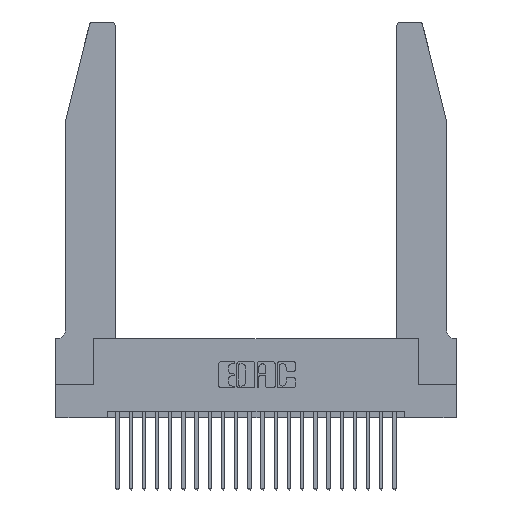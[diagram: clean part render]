
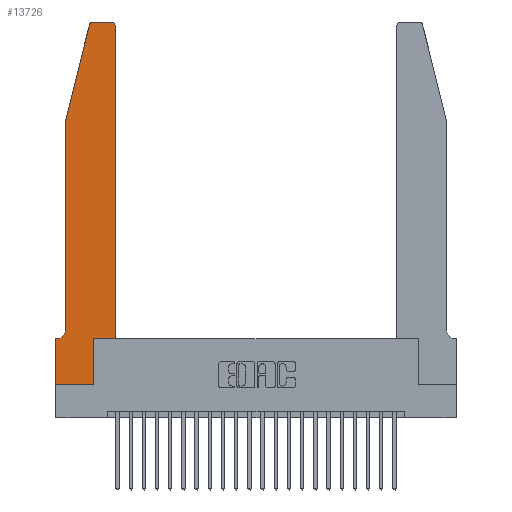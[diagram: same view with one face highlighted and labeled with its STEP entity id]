
A CAD part, top view. The second image highlights one B-rep face of the part: STEP entity #13726.
In plain terms, the highlighted planar face has unit normal (0, 0, 1).
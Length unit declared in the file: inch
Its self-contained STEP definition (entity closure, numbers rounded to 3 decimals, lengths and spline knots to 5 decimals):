
#131 = CARTESIAN_POINT ( 'NONE',  ( 0.0755, 2., 0.37 ) ) ;
#181 = CARTESIAN_POINT ( 'NONE',  ( 0., 0.35, 0.37 ) ) ;
#459 = DIRECTION ( 'NONE',  ( -1., 0., 0. ) ) ;
#518 = CARTESIAN_POINT ( 'NONE',  ( 0.0755, 2., 0.37 ) ) ;
#807 = VERTEX_POINT ( 'NONE', #22162 ) ;
#1023 = LINE ( 'NONE', #17720, #10701 ) ;
#1210 = VERTEX_POINT ( 'NONE', #16286 ) ;
#1374 = LINE ( 'NONE', #14280, #20541 ) ;
#1447 = ORIENTED_EDGE ( 'NONE', *, *, #23395, .T. ) ;
#2128 = EDGE_CURVE ( 'NONE', #6487, #19490, #15182, .T. ) ;
#2831 = VECTOR ( 'NONE', #21209, 39.37008 ) ;
#2843 = DIRECTION ( 'NONE',  ( 0., 0., 1. ) ) ;
#2980 = ORIENTED_EDGE ( 'NONE', *, *, #2128, .T. ) ;
#3807 = VECTOR ( 'NONE', #13948, 39.37008 ) ;
#4240 = DIRECTION ( 'NONE',  ( 0., -1., 0. ) ) ;
#4424 = CARTESIAN_POINT ( 'NONE',  ( 0.0055, 0.35, 0.37 ) ) ;
#5262 = ORIENTED_EDGE ( 'NONE', *, *, #6780, .T. ) ;
#5289 = VERTEX_POINT ( 'NONE', #24709 ) ;
#5668 = CIRCLE ( 'NONE', #14556, 0.03 ) ;
#5739 = VECTOR ( 'NONE', #4240, 39.37008 ) ;
#6487 = VERTEX_POINT ( 'NONE', #518 ) ;
#6617 = FACE_OUTER_BOUND ( 'NONE', #16802, .T. ) ;
#6690 = DIRECTION ( 'NONE',  ( 0., 0., 1. ) ) ;
#6777 = CARTESIAN_POINT ( 'NONE',  ( 0., 0., 0.37 ) ) ;
#6780 = EDGE_CURVE ( 'NONE', #19490, #18890, #6827, .T. ) ;
#6792 = CIRCLE ( 'NONE', #9976, 0.03 ) ;
#6824 = VERTEX_POINT ( 'NONE', #13027 ) ;
#6827 = CIRCLE ( 'NONE', #13317, 0.07 ) ;
#7191 = ORIENTED_EDGE ( 'NONE', *, *, #7594, .T. ) ;
#7594 = EDGE_CURVE ( 'NONE', #5289, #19021, #20514, .T. ) ;
#7661 = CARTESIAN_POINT ( 'NONE',  ( 0.2865, 0.35, 0.37 ) ) ;
#7665 = EDGE_CURVE ( 'NONE', #19024, #5289, #14875, .T. ) ;
#7752 = ORIENTED_EDGE ( 'NONE', *, *, #22294, .T. ) ;
#7798 = EDGE_CURVE ( 'NONE', #1210, #16410, #1023, .T. ) ;
#7847 = DIRECTION ( 'NONE',  ( 0., 0., 1. ) ) ;
#8096 = CARTESIAN_POINT ( 'NONE',  ( 0.0755, 0.42, 0.37 ) ) ;
#8776 = EDGE_CURVE ( 'NONE', #807, #6487, #20763, .T. ) ;
#9544 = VECTOR ( 'NONE', #459, 39.37008 ) ;
#9976 = AXIS2_PLACEMENT_3D ( 'NONE', #19254, #7847, #21155 ) ;
#10547 = CARTESIAN_POINT ( 'NONE',  ( 0., 0.35, 0.37 ) ) ;
#10587 = CARTESIAN_POINT ( 'NONE',  ( 0.2865, 0.35, 0.37 ) ) ;
#10701 = VECTOR ( 'NONE', #19884, 39.37008 ) ;
#10861 = LINE ( 'NONE', #23254, #5739 ) ;
#11042 = DIRECTION ( 'NONE',  ( 0., 0., -1. ) ) ;
#12054 = CARTESIAN_POINT ( 'NONE',  ( 0.4505, 0.35, 0.37 ) ) ;
#13027 = CARTESIAN_POINT ( 'NONE',  ( 0.284, 2.75, 0.37 ) ) ;
#13317 = AXIS2_PLACEMENT_3D ( 'NONE', #22405, #11042, #24312 ) ;
#13507 = EDGE_CURVE ( 'NONE', #19310, #19024, #10861, .T. ) ;
#13726 = ADVANCED_FACE ( 'NONE', ( #6617 ), #14361, .T. ) ;
#13948 = DIRECTION ( 'NONE',  ( 1., 0., 0. ) ) ;
#14006 = ORIENTED_EDGE ( 'NONE', *, *, #8776, .T. ) ;
#14280 = CARTESIAN_POINT ( 'NONE',  ( 0.0755, 0.35, 0.37 ) ) ;
#14361 = PLANE ( 'NONE',  #21544 ) ;
#14556 = AXIS2_PLACEMENT_3D ( 'NONE', #18112, #6690, #20033 ) ;
#14583 = LINE ( 'NONE', #23378, #9544 ) ;
#14875 = LINE ( 'NONE', #19301, #2831 ) ;
#14963 = EDGE_CURVE ( 'NONE', #6824, #807, #5668, .T. ) ;
#15182 = LINE ( 'NONE', #131, #24077 ) ;
#15705 = VECTOR ( 'NONE', #17114, 39.37008 ) ;
#16052 = ORIENTED_EDGE ( 'NONE', *, *, #17609, .T. ) ;
#16284 = DIRECTION ( 'NONE',  ( 1., 0., 0. ) ) ;
#16286 = CARTESIAN_POINT ( 'NONE',  ( 0.4505, 0.35, 0.37 ) ) ;
#16410 = VERTEX_POINT ( 'NONE', #22385 ) ;
#16802 = EDGE_LOOP ( 'NONE', ( #7752, #24374, #14006, #2980, #5262, #16052, #18523, #24167, #7191, #17922, #20006, #1447 ) ) ;
#17114 = DIRECTION ( 'NONE',  ( -0.239, -0.971, 0. ) ) ;
#17160 = DIRECTION ( 'NONE',  ( 0., 1., 0. ) ) ;
#17409 = DIRECTION ( 'NONE',  ( 0., -1., 0. ) ) ;
#17467 = EDGE_CURVE ( 'NONE', #19021, #1210, #19061, .T. ) ;
#17609 = EDGE_CURVE ( 'NONE', #18890, #19310, #1374, .T. ) ;
#17720 = CARTESIAN_POINT ( 'NONE',  ( 0.4505, 0.35, 0.37 ) ) ;
#17922 = ORIENTED_EDGE ( 'NONE', *, *, #17467, .T. ) ;
#18014 = DIRECTION ( 'NONE',  ( -1., 0., 0. ) ) ;
#18112 = CARTESIAN_POINT ( 'NONE',  ( 0.284, 2.72, 0.37 ) ) ;
#18523 = ORIENTED_EDGE ( 'NONE', *, *, #13507, .T. ) ;
#18890 = VERTEX_POINT ( 'NONE', #4424 ) ;
#19021 = VERTEX_POINT ( 'NONE', #10587 ) ;
#19024 = VERTEX_POINT ( 'NONE', #6777 ) ;
#19061 = LINE ( 'NONE', #12054, #3807 ) ;
#19254 = CARTESIAN_POINT ( 'NONE',  ( 0.4205, 2.72, 0.37 ) ) ;
#19301 = CARTESIAN_POINT ( 'NONE',  ( 0., 0., 0.37 ) ) ;
#19310 = VERTEX_POINT ( 'NONE', #181 ) ;
#19490 = VERTEX_POINT ( 'NONE', #8096 ) ;
#19884 = DIRECTION ( 'NONE',  ( 0., 1., 0. ) ) ;
#20006 = ORIENTED_EDGE ( 'NONE', *, *, #7798, .T. ) ;
#20033 = DIRECTION ( 'NONE',  ( 1., 0., 0. ) ) ;
#20514 = LINE ( 'NONE', #7661, #24358 ) ;
#20541 = VECTOR ( 'NONE', #18014, 39.37008 ) ;
#20763 = LINE ( 'NONE', #24639, #15705 ) ;
#21155 = DIRECTION ( 'NONE',  ( 1., 0., 0. ) ) ;
#21209 = DIRECTION ( 'NONE',  ( 1., 0., 0. ) ) ;
#21211 = CARTESIAN_POINT ( 'NONE',  ( 0.4205, 2.75, 0.37 ) ) ;
#21544 = AXIS2_PLACEMENT_3D ( 'NONE', #10547, #2843, #16284 ) ;
#21925 = VERTEX_POINT ( 'NONE', #21211 ) ;
#22162 = CARTESIAN_POINT ( 'NONE',  ( 0.25487, 2.72718, 0.37 ) ) ;
#22294 = EDGE_CURVE ( 'NONE', #21925, #6824, #14583, .T. ) ;
#22385 = CARTESIAN_POINT ( 'NONE',  ( 0.4505, 2.72, 0.37 ) ) ;
#22405 = CARTESIAN_POINT ( 'NONE',  ( 0.0055, 0.42, 0.37 ) ) ;
#23254 = CARTESIAN_POINT ( 'NONE',  ( 0., 0., 0.37 ) ) ;
#23378 = CARTESIAN_POINT ( 'NONE',  ( 0.2605, 2.75, 0.37 ) ) ;
#23395 = EDGE_CURVE ( 'NONE', #16410, #21925, #6792, .T. ) ;
#24077 = VECTOR ( 'NONE', #17409, 39.37008 ) ;
#24167 = ORIENTED_EDGE ( 'NONE', *, *, #7665, .T. ) ;
#24312 = DIRECTION ( 'NONE',  ( -1., 0., 0. ) ) ;
#24358 = VECTOR ( 'NONE', #17160, 39.37008 ) ;
#24374 = ORIENTED_EDGE ( 'NONE', *, *, #14963, .T. ) ;
#24639 = CARTESIAN_POINT ( 'NONE',  ( 0.0755, 2., 0.37 ) ) ;
#24709 = CARTESIAN_POINT ( 'NONE',  ( 0.2865, 0., 0.37 ) ) ;
